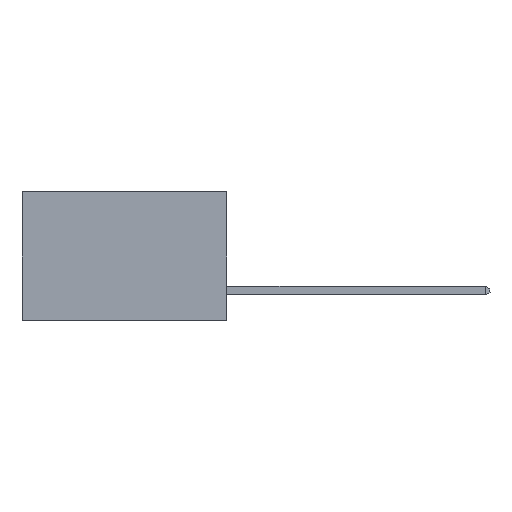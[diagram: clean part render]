
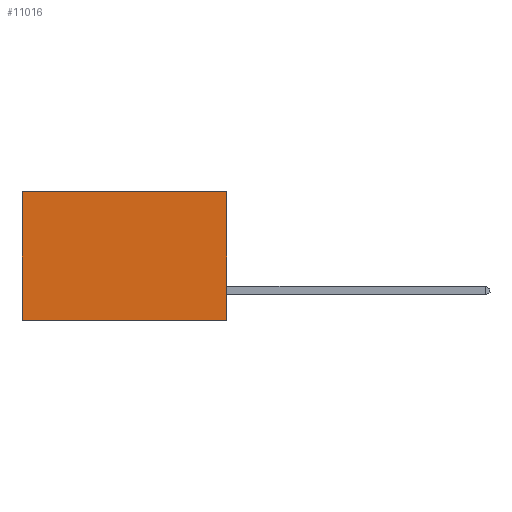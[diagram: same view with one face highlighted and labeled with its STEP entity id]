
A CAD part, left-side view. The second image highlights one B-rep face of the part: STEP entity #11016.
In plain terms, the highlighted planar face has unit normal (-1, 0, 0).
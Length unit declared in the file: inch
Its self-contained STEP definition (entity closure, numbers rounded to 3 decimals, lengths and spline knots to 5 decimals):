
#776 = LINE ( 'NONE', #8037, #15110 ) ;
#1177 = VERTEX_POINT ( 'NONE', #9488 ) ;
#1378 = LINE ( 'NONE', #9704, #10218 ) ;
#1600 = VERTEX_POINT ( 'NONE', #2463 ) ;
#1755 = FACE_OUTER_BOUND ( 'NONE', #2347, .T. ) ;
#1789 = EDGE_CURVE ( 'NONE', #10818, #1600, #13868, .T. ) ;
#1931 = EDGE_CURVE ( 'NONE', #1177, #1600, #776, .T. ) ;
#2022 = ORIENTED_EDGE ( 'NONE', *, *, #11078, .F. ) ;
#2210 = DIRECTION ( 'NONE',  ( 0., 1., 0. ) ) ;
#2347 = EDGE_LOOP ( 'NONE', ( #4465, #14313, #2022, #8772 ) ) ;
#2463 = CARTESIAN_POINT ( 'NONE',  ( 0.277, 0.59, -0.37 ) ) ;
#3629 = DIRECTION ( 'NONE',  ( 1., 0., 0. ) ) ;
#3737 = DIRECTION ( 'NONE',  ( 0., 0., -1. ) ) ;
#3861 = CARTESIAN_POINT ( 'NONE',  ( 0.277, 0., 0. ) ) ;
#4465 = ORIENTED_EDGE ( 'NONE', *, *, #1789, .T. ) ;
#6067 = CARTESIAN_POINT ( 'NONE',  ( 0.277, 0.59, -0.37 ) ) ;
#7215 = PLANE ( 'NONE',  #13337 ) ;
#7562 = VECTOR ( 'NONE', #11056, 39.37008 ) ;
#8037 = CARTESIAN_POINT ( 'NONE',  ( 0.277, 0., -0.37 ) ) ;
#8048 = CARTESIAN_POINT ( 'NONE',  ( 0.277, 0.59, 0. ) ) ;
#8772 = ORIENTED_EDGE ( 'NONE', *, *, #11856, .T. ) ;
#8878 = CARTESIAN_POINT ( 'NONE',  ( 0.277, 0., 0. ) ) ;
#9488 = CARTESIAN_POINT ( 'NONE',  ( 0.277, 0., -0.37 ) ) ;
#9704 = CARTESIAN_POINT ( 'NONE',  ( 0.277, 0., -0.37 ) ) ;
#10098 = DIRECTION ( 'NONE',  ( 0., 1., 0. ) ) ;
#10218 = VECTOR ( 'NONE', #3737, 39.37008 ) ;
#10805 = CARTESIAN_POINT ( 'NONE',  ( 0.277, 0., -0.37 ) ) ;
#10818 = VERTEX_POINT ( 'NONE', #8048 ) ;
#11016 = ADVANCED_FACE ( 'NONE', ( #1755 ), #7215, .F. ) ;
#11056 = DIRECTION ( 'NONE',  ( 0., 0., -1. ) ) ;
#11078 = EDGE_CURVE ( 'NONE', #14355, #1177, #1378, .T. ) ;
#11856 = EDGE_CURVE ( 'NONE', #14355, #10818, #15310, .T. ) ;
#11998 = DIRECTION ( 'NONE',  ( 0., 0., -1. ) ) ;
#13337 = AXIS2_PLACEMENT_3D ( 'NONE', #10805, #3629, #11998 ) ;
#13868 = LINE ( 'NONE', #6067, #7562 ) ;
#14313 = ORIENTED_EDGE ( 'NONE', *, *, #1931, .F. ) ;
#14355 = VERTEX_POINT ( 'NONE', #3861 ) ;
#14954 = VECTOR ( 'NONE', #10098, 39.37008 ) ;
#15110 = VECTOR ( 'NONE', #2210, 39.37008 ) ;
#15310 = LINE ( 'NONE', #8878, #14954 ) ;
